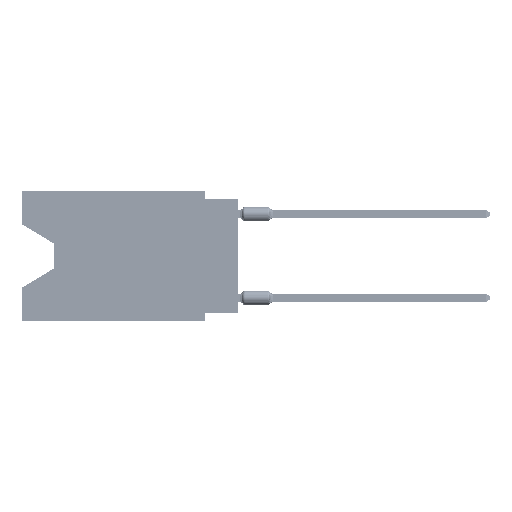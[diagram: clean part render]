
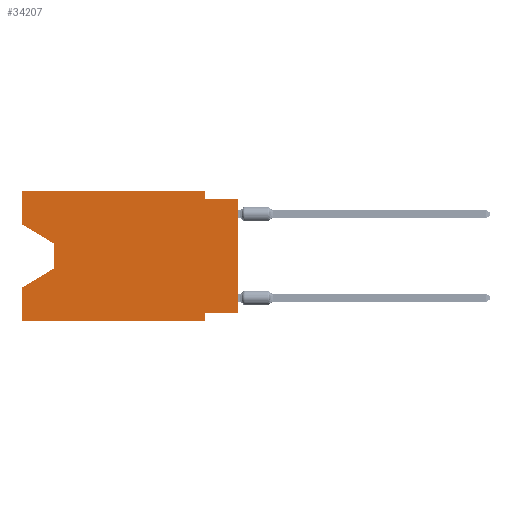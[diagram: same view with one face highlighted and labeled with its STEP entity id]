
A CAD part, left-side view. The second image highlights one B-rep face of the part: STEP entity #34207.
In plain terms, the highlighted planar face has unit normal (-1, 0, 0).
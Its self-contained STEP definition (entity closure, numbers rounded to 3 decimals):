
#306 = DIRECTION ( 'NONE',  ( 0., 0., -1. ) ) ;
#1192 = EDGE_CURVE ( 'NONE', #71092, #73806, #37117, .T. ) ;
#3004 = ORIENTED_EDGE ( 'NONE', *, *, #72490, .F. ) ;
#4899 = LINE ( 'NONE', #76321, #34302 ) ;
#7089 = CARTESIAN_POINT ( 'NONE',  ( 0., 13.97, -4.013 ) ) ;
#8214 = DIRECTION ( 'NONE',  ( 1., 0., 0. ) ) ;
#9890 = CARTESIAN_POINT ( 'NONE',  ( 0., 0., 0. ) ) ;
#10246 = LINE ( 'NONE', #16607, #66329 ) ;
#13799 = DIRECTION ( 'NONE',  ( 0., 0., -1. ) ) ;
#14251 = VECTOR ( 'NONE', #47348, 1000. ) ;
#15020 = ORIENTED_EDGE ( 'NONE', *, *, #24799, .F. ) ;
#15169 = CARTESIAN_POINT ( 'NONE',  ( 0., 16.383, -9.906 ) ) ;
#16417 = DIRECTION ( 'NONE',  ( 0., 0., 1. ) ) ;
#16607 = CARTESIAN_POINT ( 'NONE',  ( 0., 0., -0.635 ) ) ;
#16908 = CARTESIAN_POINT ( 'NONE',  ( 0., 0., -9.271 ) ) ;
#17180 = CARTESIAN_POINT ( 'NONE',  ( 0., 2.54, 0. ) ) ;
#17710 = EDGE_CURVE ( 'NONE', #58818, #42545, #60227, .T. ) ;
#18672 = DIRECTION ( 'NONE',  ( 0., 0., -1. ) ) ;
#21549 = VECTOR ( 'NONE', #16417, 1000. ) ;
#22911 = LINE ( 'NONE', #16908, #53053 ) ;
#23371 = LINE ( 'NONE', #47741, #14251 ) ;
#23756 = CARTESIAN_POINT ( 'NONE',  ( 0., 13.97, -5.893 ) ) ;
#23888 = CARTESIAN_POINT ( 'NONE',  ( 0., 2.54, -0.635 ) ) ;
#24215 = CARTESIAN_POINT ( 'NONE',  ( 0., 16.383, -2.546 ) ) ;
#24275 = CARTESIAN_POINT ( 'NONE',  ( 0., 16.383, 0. ) ) ;
#24799 = EDGE_CURVE ( 'NONE', #62070, #58818, #22911, .T. ) ;
#25438 = LINE ( 'NONE', #7089, #72261 ) ;
#26384 = ORIENTED_EDGE ( 'NONE', *, *, #71826, .F. ) ;
#30522 = VECTOR ( 'NONE', #59547, 1000. ) ;
#33742 = VECTOR ( 'NONE', #37907, 1000. ) ;
#33846 = LINE ( 'NONE', #9890, #58262 ) ;
#34207 = ADVANCED_FACE ( 'NONE', ( #44547 ), #44162, .F. ) ;
#34302 = VECTOR ( 'NONE', #58389, 1000. ) ;
#34308 = ORIENTED_EDGE ( 'NONE', *, *, #17710, .F. ) ;
#34493 = LINE ( 'NONE', #53245, #45836 ) ;
#35119 = VERTEX_POINT ( 'NONE', #15169 ) ;
#35210 = CARTESIAN_POINT ( 'NONE',  ( 0., 16.383, -9.906 ) ) ;
#36464 = DIRECTION ( 'NONE',  ( 0., 0., 1. ) ) ;
#37117 = LINE ( 'NONE', #68207, #33742 ) ;
#37907 = DIRECTION ( 'NONE',  ( 0., -0.855, -0.519 ) ) ;
#38635 = ORIENTED_EDGE ( 'NONE', *, *, #42641, .T. ) ;
#39633 = ORIENTED_EDGE ( 'NONE', *, *, #59241, .T. ) ;
#39759 = VERTEX_POINT ( 'NONE', #17180 ) ;
#40363 = CARTESIAN_POINT ( 'NONE',  ( 0., 16.383, -7.36 ) ) ;
#41981 = LINE ( 'NONE', #52771, #21549 ) ;
#42545 = VERTEX_POINT ( 'NONE', #76823 ) ;
#42641 = EDGE_CURVE ( 'NONE', #75995, #65525, #59686, .T. ) ;
#43091 = CARTESIAN_POINT ( 'NONE',  ( 0., 2.54, -9.271 ) ) ;
#44162 = PLANE ( 'NONE',  #70727 ) ;
#44547 = FACE_OUTER_BOUND ( 'NONE', #76083, .T. ) ;
#45836 = VECTOR ( 'NONE', #36464, 1000. ) ;
#46233 = DIRECTION ( 'NONE',  ( 0., 0., 1. ) ) ;
#47283 = DIRECTION ( 'NONE',  ( 0., 1., 0. ) ) ;
#47348 = DIRECTION ( 'NONE',  ( 0., -1., 0. ) ) ;
#47379 = DIRECTION ( 'NONE',  ( 0., -1., 0. ) ) ;
#47741 = CARTESIAN_POINT ( 'NONE',  ( 0., 16.383, 0. ) ) ;
#48092 = EDGE_CURVE ( 'NONE', #39759, #52254, #4899, .T. ) ;
#49864 = EDGE_CURVE ( 'NONE', #60498, #39759, #23371, .T. ) ;
#52254 = VERTEX_POINT ( 'NONE', #23888 ) ;
#52464 = ORIENTED_EDGE ( 'NONE', *, *, #71831, .T. ) ;
#52771 = CARTESIAN_POINT ( 'NONE',  ( 0., 16.383, 0. ) ) ;
#53053 = VECTOR ( 'NONE', #47283, 1000. ) ;
#53245 = CARTESIAN_POINT ( 'NONE',  ( 0., 16.383, 0. ) ) ;
#53307 = DIRECTION ( 'NONE',  ( 0., 0.855, -0.519 ) ) ;
#53855 = VERTEX_POINT ( 'NONE', #78582 ) ;
#57525 = CARTESIAN_POINT ( 'NONE',  ( 0., 0., -9.271 ) ) ;
#57695 = CARTESIAN_POINT ( 'NONE',  ( 0., 16.383, 0. ) ) ;
#57775 = EDGE_CURVE ( 'NONE', #62070, #53855, #33846, .T. ) ;
#58262 = VECTOR ( 'NONE', #46233, 1000. ) ;
#58389 = DIRECTION ( 'NONE',  ( 0., 0., -1. ) ) ;
#58818 = VERTEX_POINT ( 'NONE', #43091 ) ;
#59241 = EDGE_CURVE ( 'NONE', #73806, #75995, #25438, .T. ) ;
#59547 = DIRECTION ( 'NONE',  ( 0., -1., 0. ) ) ;
#59686 = LINE ( 'NONE', #23756, #77248 ) ;
#60227 = LINE ( 'NONE', #66977, #77784 ) ;
#60498 = VERTEX_POINT ( 'NONE', #24275 ) ;
#60641 = ORIENTED_EDGE ( 'NONE', *, *, #73263, .F. ) ;
#62070 = VERTEX_POINT ( 'NONE', #57525 ) ;
#62858 = ORIENTED_EDGE ( 'NONE', *, *, #57775, .T. ) ;
#63464 = ORIENTED_EDGE ( 'NONE', *, *, #1192, .T. ) ;
#65525 = VERTEX_POINT ( 'NONE', #40363 ) ;
#66329 = VECTOR ( 'NONE', #47379, 1000. ) ;
#66977 = CARTESIAN_POINT ( 'NONE',  ( 0., 2.54, -9.906 ) ) ;
#68207 = CARTESIAN_POINT ( 'NONE',  ( 0., 16.383, -2.546 ) ) ;
#70727 = AXIS2_PLACEMENT_3D ( 'NONE', #57695, #8214, #13799 ) ;
#71092 = VERTEX_POINT ( 'NONE', #24215 ) ;
#71412 = CARTESIAN_POINT ( 'NONE',  ( 0., 13.97, -5.893 ) ) ;
#71826 = EDGE_CURVE ( 'NONE', #71092, #60498, #41981, .T. ) ;
#71831 = EDGE_CURVE ( 'NONE', #35119, #42545, #77873, .T. ) ;
#72261 = VECTOR ( 'NONE', #306, 1000. ) ;
#72378 = CARTESIAN_POINT ( 'NONE',  ( 0., 13.97, -4.013 ) ) ;
#72490 = EDGE_CURVE ( 'NONE', #35119, #65525, #34493, .T. ) ;
#73263 = EDGE_CURVE ( 'NONE', #52254, #53855, #10246, .T. ) ;
#73631 = ORIENTED_EDGE ( 'NONE', *, *, #49864, .F. ) ;
#73806 = VERTEX_POINT ( 'NONE', #72378 ) ;
#75995 = VERTEX_POINT ( 'NONE', #71412 ) ;
#76083 = EDGE_LOOP ( 'NONE', ( #63464, #39633, #38635, #3004, #52464, #34308, #15020, #62858, #60641, #76779, #73631, #26384 ) ) ;
#76321 = CARTESIAN_POINT ( 'NONE',  ( 0., 2.54, 0. ) ) ;
#76779 = ORIENTED_EDGE ( 'NONE', *, *, #48092, .F. ) ;
#76823 = CARTESIAN_POINT ( 'NONE',  ( 0., 2.54, -9.906 ) ) ;
#77248 = VECTOR ( 'NONE', #53307, 1000. ) ;
#77784 = VECTOR ( 'NONE', #18672, 1000. ) ;
#77873 = LINE ( 'NONE', #35210, #30522 ) ;
#78582 = CARTESIAN_POINT ( 'NONE',  ( 0., 0., -0.635 ) ) ;
